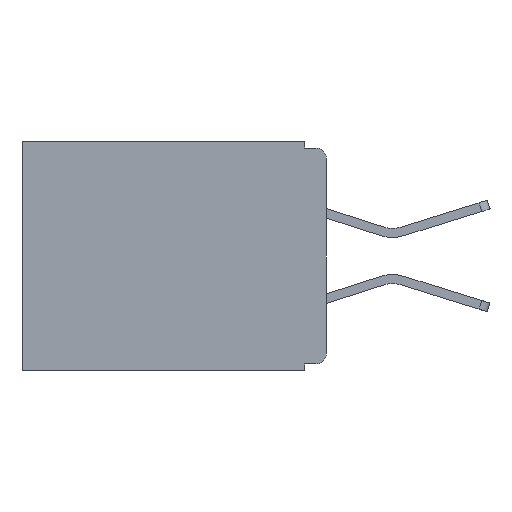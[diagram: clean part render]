
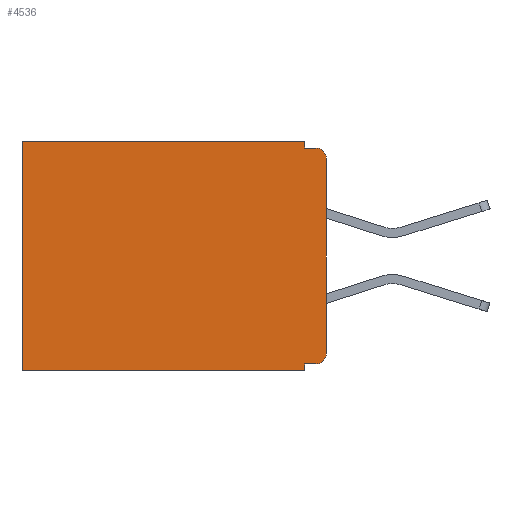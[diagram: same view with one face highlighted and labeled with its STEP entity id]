
A CAD part, left-side view. The second image highlights one B-rep face of the part: STEP entity #4536.
In plain terms, the highlighted planar face has unit normal (-1, 0, 0).
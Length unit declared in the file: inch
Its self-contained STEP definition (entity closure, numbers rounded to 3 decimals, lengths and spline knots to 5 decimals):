
#135 = CARTESIAN_POINT ( 'NONE',  ( 0.3, 0.031, -0.33 ) ) ;
#392 = DIRECTION ( 'NONE',  ( 0., 0., -1. ) ) ;
#883 = VERTEX_POINT ( 'NONE', #14709 ) ;
#1148 = EDGE_CURVE ( 'NONE', #11792, #10441, #17455, .T. ) ;
#1195 = DIRECTION ( 'NONE',  ( 0., 1., 0. ) ) ;
#1240 = VERTEX_POINT ( 'NONE', #4346 ) ;
#1519 = CARTESIAN_POINT ( 'NONE',  ( 0.3, 0.437, -0.33 ) ) ;
#1677 = ORIENTED_EDGE ( 'NONE', *, *, #5224, .T. ) ;
#1806 = VERTEX_POINT ( 'NONE', #16584 ) ;
#2713 = DIRECTION ( 'NONE',  ( 0., 1., 0. ) ) ;
#3224 = CARTESIAN_POINT ( 'NONE',  ( 0.3, 0.015, -0.305 ) ) ;
#3420 = VECTOR ( 'NONE', #2713, 39.37008 ) ;
#3431 = EDGE_CURVE ( 'NONE', #17186, #11792, #19053, .T. ) ;
#3461 = LINE ( 'NONE', #15744, #8995 ) ;
#3701 = EDGE_CURVE ( 'NONE', #883, #18292, #3461, .T. ) ;
#3773 = CARTESIAN_POINT ( 'NONE',  ( 0.3, 0.437, -0.33 ) ) ;
#3977 = LINE ( 'NONE', #21135, #3420 ) ;
#4059 = CARTESIAN_POINT ( 'NONE',  ( 0.3, 0., -0.305 ) ) ;
#4346 = CARTESIAN_POINT ( 'NONE',  ( 0.3, 0., -0.025 ) ) ;
#4536 = ADVANCED_FACE ( 'NONE', ( #19907 ), #7063, .F. ) ;
#4817 = ORIENTED_EDGE ( 'NONE', *, *, #18724, .T. ) ;
#5067 = DIRECTION ( 'NONE',  ( 0., 0., -1. ) ) ;
#5152 = LINE ( 'NONE', #3773, #9512 ) ;
#5224 = EDGE_CURVE ( 'NONE', #20803, #11928, #5152, .T. ) ;
#5598 = EDGE_CURVE ( 'NONE', #1806, #11928, #6868, .T. ) ;
#5810 = ORIENTED_EDGE ( 'NONE', *, *, #13986, .F. ) ;
#5937 = CARTESIAN_POINT ( 'NONE',  ( 0.3, 0.031, 0. ) ) ;
#6797 = ORIENTED_EDGE ( 'NONE', *, *, #22204, .F. ) ;
#6868 = LINE ( 'NONE', #21598, #15543 ) ;
#7063 = PLANE ( 'NONE',  #23285 ) ;
#8247 = EDGE_CURVE ( 'NONE', #1240, #10441, #17505, .T. ) ;
#8995 = VECTOR ( 'NONE', #20756, 39.37008 ) ;
#9280 = VECTOR ( 'NONE', #13659, 39.37008 ) ;
#9512 = VECTOR ( 'NONE', #11200, 39.37008 ) ;
#9610 = CARTESIAN_POINT ( 'NONE',  ( 0.3, 0., -0.33 ) ) ;
#10044 = LINE ( 'NONE', #135, #14377 ) ;
#10441 = VERTEX_POINT ( 'NONE', #23236 ) ;
#11200 = DIRECTION ( 'NONE',  ( 0., 0., -1. ) ) ;
#11446 = ORIENTED_EDGE ( 'NONE', *, *, #3431, .F. ) ;
#11634 = ORIENTED_EDGE ( 'NONE', *, *, #16477, .T. ) ;
#11792 = VERTEX_POINT ( 'NONE', #20520 ) ;
#11797 = CARTESIAN_POINT ( 'NONE',  ( 0.3, 0., -0.01 ) ) ;
#11843 = DIRECTION ( 'NONE',  ( 0., 0., -1. ) ) ;
#11928 = VERTEX_POINT ( 'NONE', #1519 ) ;
#12097 = DIRECTION ( 'NONE',  ( 1., 0., 0. ) ) ;
#12302 = ORIENTED_EDGE ( 'NONE', *, *, #8247, .T. ) ;
#12584 = VECTOR ( 'NONE', #14256, 39.37008 ) ;
#13659 = DIRECTION ( 'NONE',  ( 0., 0., -1. ) ) ;
#13986 = EDGE_CURVE ( 'NONE', #18292, #1806, #10044, .T. ) ;
#14223 = LINE ( 'NONE', #9610, #23344 ) ;
#14256 = DIRECTION ( 'NONE',  ( 0., -1., 0. ) ) ;
#14377 = VECTOR ( 'NONE', #14885, 39.37008 ) ;
#14515 = CARTESIAN_POINT ( 'NONE',  ( 0.3, 0.031, 0. ) ) ;
#14709 = CARTESIAN_POINT ( 'NONE',  ( 0.3, 0.015, -0.32 ) ) ;
#14885 = DIRECTION ( 'NONE',  ( 0., 0., -1. ) ) ;
#15543 = VECTOR ( 'NONE', #1195, 39.37008 ) ;
#15665 = ORIENTED_EDGE ( 'NONE', *, *, #3701, .F. ) ;
#15744 = CARTESIAN_POINT ( 'NONE',  ( 0.3, 0., -0.32 ) ) ;
#16148 = DIRECTION ( 'NONE',  ( -1., 0., 0. ) ) ;
#16477 = EDGE_CURVE ( 'NONE', #883, #22837, #19406, .T. ) ;
#16584 = CARTESIAN_POINT ( 'NONE',  ( 0.3, 0.031, -0.33 ) ) ;
#16894 = DIRECTION ( 'NONE',  ( -1., 0., 0. ) ) ;
#16896 = CARTESIAN_POINT ( 'NONE',  ( 0.3, 0.015, -0.025 ) ) ;
#17094 = DIRECTION ( 'NONE',  ( 0., 0., -1. ) ) ;
#17186 = VERTEX_POINT ( 'NONE', #14515 ) ;
#17455 = LINE ( 'NONE', #11797, #12584 ) ;
#17505 = CIRCLE ( 'NONE', #23496, 0.015 ) ;
#17716 = AXIS2_PLACEMENT_3D ( 'NONE', #3224, #16148, #5067 ) ;
#18292 = VERTEX_POINT ( 'NONE', #21699 ) ;
#18724 = EDGE_CURVE ( 'NONE', #17186, #20803, #3977, .T. ) ;
#19053 = LINE ( 'NONE', #5937, #9280 ) ;
#19309 = ORIENTED_EDGE ( 'NONE', *, *, #5598, .F. ) ;
#19406 = CIRCLE ( 'NONE', #17716, 0.015 ) ;
#19515 = ORIENTED_EDGE ( 'NONE', *, *, #1148, .F. ) ;
#19907 = FACE_OUTER_BOUND ( 'NONE', #20295, .T. ) ;
#20295 = EDGE_LOOP ( 'NONE', ( #6797, #12302, #19515, #11446, #4817, #1677, #19309, #5810, #15665, #11634 ) ) ;
#20520 = CARTESIAN_POINT ( 'NONE',  ( 0.3, 0.031, -0.01 ) ) ;
#20756 = DIRECTION ( 'NONE',  ( 0., 1., 0. ) ) ;
#20803 = VERTEX_POINT ( 'NONE', #21835 ) ;
#21135 = CARTESIAN_POINT ( 'NONE',  ( 0.3, 0., 0. ) ) ;
#21598 = CARTESIAN_POINT ( 'NONE',  ( 0.3, 0., -0.33 ) ) ;
#21699 = CARTESIAN_POINT ( 'NONE',  ( 0.3, 0.031, -0.32 ) ) ;
#21835 = CARTESIAN_POINT ( 'NONE',  ( 0.3, 0.437, 0. ) ) ;
#22204 = EDGE_CURVE ( 'NONE', #1240, #22837, #14223, .T. ) ;
#22386 = CARTESIAN_POINT ( 'NONE',  ( 0.3, 0., -0.33 ) ) ;
#22837 = VERTEX_POINT ( 'NONE', #4059 ) ;
#23236 = CARTESIAN_POINT ( 'NONE',  ( 0.3, 0.015, -0.01 ) ) ;
#23285 = AXIS2_PLACEMENT_3D ( 'NONE', #22386, #12097, #11843 ) ;
#23344 = VECTOR ( 'NONE', #392, 39.37008 ) ;
#23496 = AXIS2_PLACEMENT_3D ( 'NONE', #16896, #16894, #17094 ) ;
